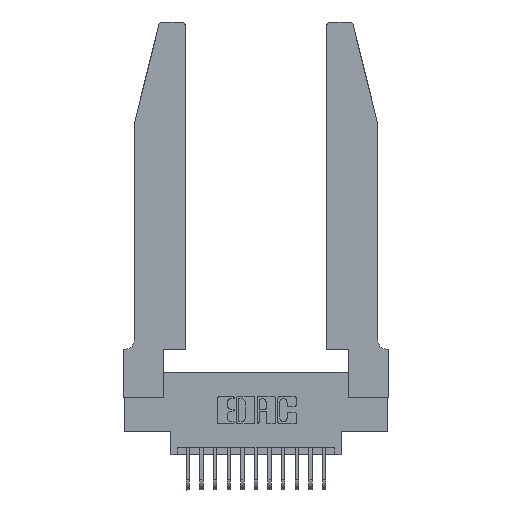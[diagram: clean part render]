
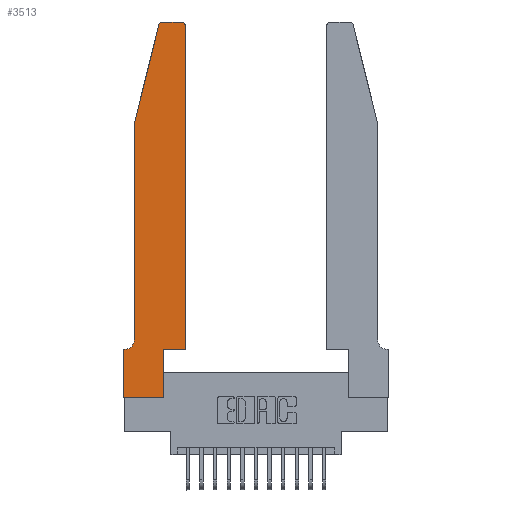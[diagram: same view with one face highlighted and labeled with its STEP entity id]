
A CAD part, top view. The second image highlights one B-rep face of the part: STEP entity #3513.
In plain terms, the highlighted planar face has unit normal (0, 0, 1).
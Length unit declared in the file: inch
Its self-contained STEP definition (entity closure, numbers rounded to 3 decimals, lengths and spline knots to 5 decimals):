
#20 = LINE ( 'NONE', #11290, #3219 ) ;
#40 = CARTESIAN_POINT ( 'NONE',  ( 0.4505, 0.35, 0.37 ) ) ;
#245 = LINE ( 'NONE', #5859, #6180 ) ;
#489 = CARTESIAN_POINT ( 'NONE',  ( 0.4505, 2.72, 0.37 ) ) ;
#537 = VECTOR ( 'NONE', #2190, 39.37008 ) ;
#957 = LINE ( 'NONE', #12564, #11297 ) ;
#1106 = EDGE_CURVE ( 'NONE', #5986, #8467, #13460, .T. ) ;
#1703 = AXIS2_PLACEMENT_3D ( 'NONE', #14359, #6309, #15713 ) ;
#1740 = DIRECTION ( 'NONE',  ( 0., -1., 0. ) ) ;
#1764 = EDGE_CURVE ( 'NONE', #14713, #15393, #6928, .T. ) ;
#2017 = CARTESIAN_POINT ( 'NONE',  ( 0.284, 2.72, 0.37 ) ) ;
#2105 = CARTESIAN_POINT ( 'NONE',  ( 0.4505, 0.35, 0.37 ) ) ;
#2190 = DIRECTION ( 'NONE',  ( 0., 1., 0. ) ) ;
#2651 = ORIENTED_EDGE ( 'NONE', *, *, #11722, .T. ) ;
#2778 = ORIENTED_EDGE ( 'NONE', *, *, #1106, .T. ) ;
#3070 = ORIENTED_EDGE ( 'NONE', *, *, #10115, .T. ) ;
#3156 = CARTESIAN_POINT ( 'NONE',  ( 0.2865, 0.35, 0.37 ) ) ;
#3219 = VECTOR ( 'NONE', #5941, 39.37008 ) ;
#3396 = DIRECTION ( 'NONE',  ( 1., 0., 0. ) ) ;
#3513 = ADVANCED_FACE ( 'NONE', ( #7084 ), #13973, .T. ) ;
#3612 = CARTESIAN_POINT ( 'NONE',  ( 0., 0.35, 0.37 ) ) ;
#3952 = CARTESIAN_POINT ( 'NONE',  ( 0., 0., 0.37 ) ) ;
#4230 = CARTESIAN_POINT ( 'NONE',  ( 0.0755, 0.42, 0.37 ) ) ;
#4532 = EDGE_CURVE ( 'NONE', #15688, #10657, #17122, .T. ) ;
#4550 = CARTESIAN_POINT ( 'NONE',  ( 0., 0.35, 0.37 ) ) ;
#4711 = CARTESIAN_POINT ( 'NONE',  ( 0.0755, 2., 0.37 ) ) ;
#4917 = CARTESIAN_POINT ( 'NONE',  ( 0.0055, 0.35, 0.37 ) ) ;
#4999 = LINE ( 'NONE', #12988, #537 ) ;
#5438 = ORIENTED_EDGE ( 'NONE', *, *, #14526, .T. ) ;
#5860 = DIRECTION ( 'NONE',  ( -1., 0., 0. ) ) ;
#5859 = CARTESIAN_POINT ( 'NONE',  ( 0.2605, 2.75, 0.37 ) ) ;
#5908 = DIRECTION ( 'NONE',  ( 0., 0., 1. ) ) ;
#5941 = DIRECTION ( 'NONE',  ( 1., 0., 0. ) ) ;
#5986 = VERTEX_POINT ( 'NONE', #6147 ) ;
#6147 = CARTESIAN_POINT ( 'NONE',  ( 0.2865, 0., 0.37 ) ) ;
#6180 = VECTOR ( 'NONE', #12683, 39.37008 ) ;
#6263 = VERTEX_POINT ( 'NONE', #16110 ) ;
#6288 = LINE ( 'NONE', #2105, #16565 ) ;
#6309 = DIRECTION ( 'NONE',  ( 0., 0., 1. ) ) ;
#6328 = LINE ( 'NONE', #7304, #7198 ) ;
#6594 = CARTESIAN_POINT ( 'NONE',  ( 0.0055, 0.42, 0.37 ) ) ;
#6787 = EDGE_CURVE ( 'NONE', #17305, #7334, #11391, .T. ) ;
#6928 = LINE ( 'NONE', #12551, #10084 ) ;
#7084 = FACE_OUTER_BOUND ( 'NONE', #9756, .T. ) ;
#7133 = EDGE_CURVE ( 'NONE', #6263, #12050, #6328, .T. ) ;
#7198 = VECTOR ( 'NONE', #8653, 39.37008 ) ;
#7304 = CARTESIAN_POINT ( 'NONE',  ( 0.0755, 2., 0.37 ) ) ;
#7334 = VERTEX_POINT ( 'NONE', #4917 ) ;
#7863 = AXIS2_PLACEMENT_3D ( 'NONE', #6594, #15985, #7946 ) ;
#7946 = DIRECTION ( 'NONE',  ( -1., 0., 0. ) ) ;
#7981 = ORIENTED_EDGE ( 'NONE', *, *, #6787, .T. ) ;
#8467 = VERTEX_POINT ( 'NONE', #12654 ) ;
#8653 = DIRECTION ( 'NONE',  ( -0.239, -0.971, 0. ) ) ;
#9141 = ORIENTED_EDGE ( 'NONE', *, *, #1764, .T. ) ;
#9490 = VECTOR ( 'NONE', #11221, 39.37008 ) ;
#9756 = EDGE_LOOP ( 'NONE', ( #5438, #2651, #13745, #14548, #7981, #14313, #9141, #9946, #2778, #3070, #12312, #13623 ) ) ;
#9946 = ORIENTED_EDGE ( 'NONE', *, *, #13997, .T. ) ;
#10029 = CIRCLE ( 'NONE', #16442, 0.03 ) ;
#10084 = VECTOR ( 'NONE', #1740, 39.37008 ) ;
#10115 = EDGE_CURVE ( 'NONE', #8467, #11610, #6288, .T. ) ;
#10210 = DIRECTION ( 'NONE',  ( 1., 0., 0. ) ) ;
#10647 = LINE ( 'NONE', #4711, #13795 ) ;
#10657 = VERTEX_POINT ( 'NONE', #11573 ) ;
#10701 = EDGE_CURVE ( 'NONE', #11610, #15688, #4999, .T. ) ;
#11142 = EDGE_CURVE ( 'NONE', #7334, #14713, #957, .T. ) ;
#11221 = DIRECTION ( 'NONE',  ( 0., 1., 0. ) ) ;
#11290 = CARTESIAN_POINT ( 'NONE',  ( 0., 0., 0.37 ) ) ;
#11297 = VECTOR ( 'NONE', #5860, 39.37008 ) ;
#11391 = CIRCLE ( 'NONE', #7863, 0.07 ) ;
#11451 = DIRECTION ( 'NONE',  ( 0., 0., 1. ) ) ;
#11573 = CARTESIAN_POINT ( 'NONE',  ( 0.4205, 2.75, 0.37 ) ) ;
#11610 = VERTEX_POINT ( 'NONE', #40 ) ;
#11722 = EDGE_CURVE ( 'NONE', #12209, #6263, #10029, .T. ) ;
#12050 = VERTEX_POINT ( 'NONE', #12268 ) ;
#12209 = VERTEX_POINT ( 'NONE', #16771 ) ;
#12268 = CARTESIAN_POINT ( 'NONE',  ( 0.0755, 2., 0.37 ) ) ;
#12312 = ORIENTED_EDGE ( 'NONE', *, *, #10701, .T. ) ;
#12551 = CARTESIAN_POINT ( 'NONE',  ( 0., 0., 0.37 ) ) ;
#12564 = CARTESIAN_POINT ( 'NONE',  ( 0.0755, 0.35, 0.37 ) ) ;
#12654 = CARTESIAN_POINT ( 'NONE',  ( 0.2865, 0.35, 0.37 ) ) ;
#12683 = DIRECTION ( 'NONE',  ( -1., 0., 0. ) ) ;
#12820 = EDGE_CURVE ( 'NONE', #12050, #17305, #10647, .T. ) ;
#12988 = CARTESIAN_POINT ( 'NONE',  ( 0.4505, 0.35, 0.37 ) ) ;
#13004 = AXIS2_PLACEMENT_3D ( 'NONE', #4550, #5908, #15311 ) ;
#13460 = LINE ( 'NONE', #3156, #9490 ) ;
#13623 = ORIENTED_EDGE ( 'NONE', *, *, #4532, .T. ) ;
#13745 = ORIENTED_EDGE ( 'NONE', *, *, #7133, .T. ) ;
#13795 = VECTOR ( 'NONE', #15471, 39.37008 ) ;
#13973 = PLANE ( 'NONE',  #13004 ) ;
#13997 = EDGE_CURVE ( 'NONE', #15393, #5986, #20, .T. ) ;
#14313 = ORIENTED_EDGE ( 'NONE', *, *, #11142, .T. ) ;
#14359 = CARTESIAN_POINT ( 'NONE',  ( 0.4205, 2.72, 0.37 ) ) ;
#14526 = EDGE_CURVE ( 'NONE', #10657, #12209, #245, .T. ) ;
#14548 = ORIENTED_EDGE ( 'NONE', *, *, #12820, .T. ) ;
#14713 = VERTEX_POINT ( 'NONE', #3612 ) ;
#15311 = DIRECTION ( 'NONE',  ( 1., 0., 0. ) ) ;
#15393 = VERTEX_POINT ( 'NONE', #3952 ) ;
#15471 = DIRECTION ( 'NONE',  ( 0., -1., 0. ) ) ;
#15688 = VERTEX_POINT ( 'NONE', #489 ) ;
#15713 = DIRECTION ( 'NONE',  ( 1., 0., 0. ) ) ;
#15985 = DIRECTION ( 'NONE',  ( 0., 0., -1. ) ) ;
#16110 = CARTESIAN_POINT ( 'NONE',  ( 0.25487, 2.72718, 0.37 ) ) ;
#16442 = AXIS2_PLACEMENT_3D ( 'NONE', #2017, #11451, #3396 ) ;
#16565 = VECTOR ( 'NONE', #10210, 39.37008 ) ;
#16771 = CARTESIAN_POINT ( 'NONE',  ( 0.284, 2.75, 0.37 ) ) ;
#17122 = CIRCLE ( 'NONE', #1703, 0.03 ) ;
#17305 = VERTEX_POINT ( 'NONE', #4230 ) ;
